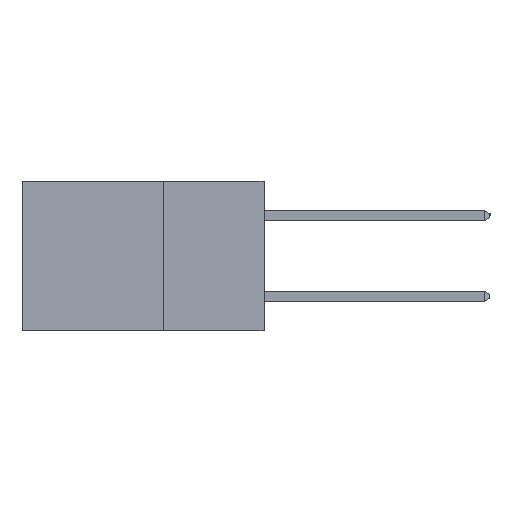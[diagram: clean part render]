
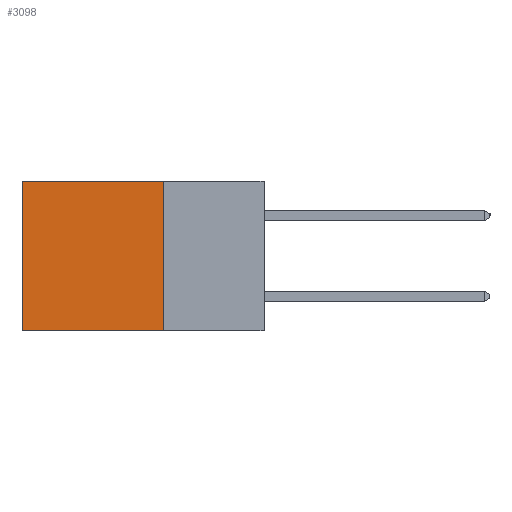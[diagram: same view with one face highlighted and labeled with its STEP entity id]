
A CAD part, left-side view. The second image highlights one B-rep face of the part: STEP entity #3098.
In plain terms, the highlighted planar face has unit normal (-1, 0, 0).
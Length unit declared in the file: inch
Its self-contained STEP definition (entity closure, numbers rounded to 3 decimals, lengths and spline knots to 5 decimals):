
#84 = CARTESIAN_POINT ( 'NONE',  ( 0.2615, 0.25, -0.37 ) ) ;
#540 = EDGE_CURVE ( 'NONE', #13805, #12658, #10293, .T. ) ;
#703 = VECTOR ( 'NONE', #2245, 39.37008 ) ;
#1024 = DIRECTION ( 'NONE',  ( 1., 0., 0. ) ) ;
#1251 = DIRECTION ( 'NONE',  ( 0., 0., -1. ) ) ;
#2245 = DIRECTION ( 'NONE',  ( 0., 1., 0. ) ) ;
#2712 = CARTESIAN_POINT ( 'NONE',  ( 0.2615, 0.6, 0. ) ) ;
#3098 = ADVANCED_FACE ( 'NONE', ( #14055 ), #10347, .F. ) ;
#3901 = VERTEX_POINT ( 'NONE', #13896 ) ;
#4044 = EDGE_CURVE ( 'NONE', #14063, #3901, #13171, .T. ) ;
#4117 = DIRECTION ( 'NONE',  ( 0., 1., 0. ) ) ;
#4208 = EDGE_CURVE ( 'NONE', #3901, #12658, #13491, .T. ) ;
#4653 = LINE ( 'NONE', #5852, #703 ) ;
#5388 = VECTOR ( 'NONE', #4117, 39.37008 ) ;
#5852 = CARTESIAN_POINT ( 'NONE',  ( 0.2615, 0.25, 0. ) ) ;
#6479 = CARTESIAN_POINT ( 'NONE',  ( 0.2615, 0.6, -0.37 ) ) ;
#6491 = CARTESIAN_POINT ( 'NONE',  ( 0.2615, 0.25, -0.37 ) ) ;
#7054 = EDGE_CURVE ( 'NONE', #14063, #13805, #4653, .T. ) ;
#7789 = EDGE_LOOP ( 'NONE', ( #12939, #9435, #13147, #10704 ) ) ;
#9046 = AXIS2_PLACEMENT_3D ( 'NONE', #13970, #1024, #13892 ) ;
#9435 = ORIENTED_EDGE ( 'NONE', *, *, #4208, .F. ) ;
#10221 = CARTESIAN_POINT ( 'NONE',  ( 0.2615, 0.6, -0.37 ) ) ;
#10293 = LINE ( 'NONE', #10221, #12255 ) ;
#10347 = PLANE ( 'NONE',  #9046 ) ;
#10704 = ORIENTED_EDGE ( 'NONE', *, *, #7054, .T. ) ;
#12255 = VECTOR ( 'NONE', #14948, 39.37008 ) ;
#12658 = VERTEX_POINT ( 'NONE', #6479 ) ;
#12939 = ORIENTED_EDGE ( 'NONE', *, *, #540, .T. ) ;
#13147 = ORIENTED_EDGE ( 'NONE', *, *, #4044, .F. ) ;
#13171 = LINE ( 'NONE', #84, #14356 ) ;
#13491 = LINE ( 'NONE', #6491, #5388 ) ;
#13805 = VERTEX_POINT ( 'NONE', #2712 ) ;
#13892 = DIRECTION ( 'NONE',  ( 0., 0., -1. ) ) ;
#13896 = CARTESIAN_POINT ( 'NONE',  ( 0.2615, 0.25, -0.37 ) ) ;
#13970 = CARTESIAN_POINT ( 'NONE',  ( 0.2615, 0.25, -0.37 ) ) ;
#14055 = FACE_OUTER_BOUND ( 'NONE', #7789, .T. ) ;
#14063 = VERTEX_POINT ( 'NONE', #14436 ) ;
#14356 = VECTOR ( 'NONE', #1251, 39.37008 ) ;
#14436 = CARTESIAN_POINT ( 'NONE',  ( 0.2615, 0.25, 0. ) ) ;
#14948 = DIRECTION ( 'NONE',  ( 0., 0., -1. ) ) ;
